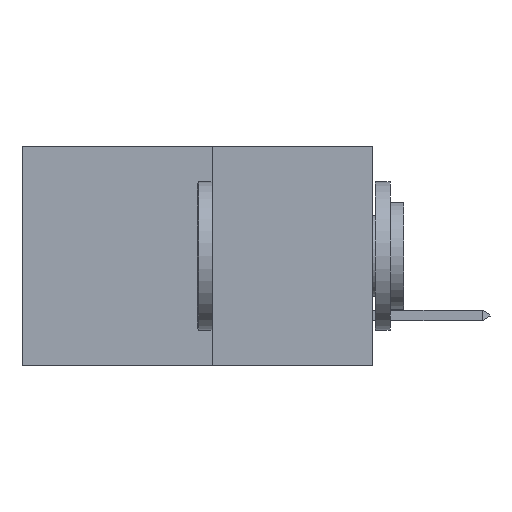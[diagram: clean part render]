
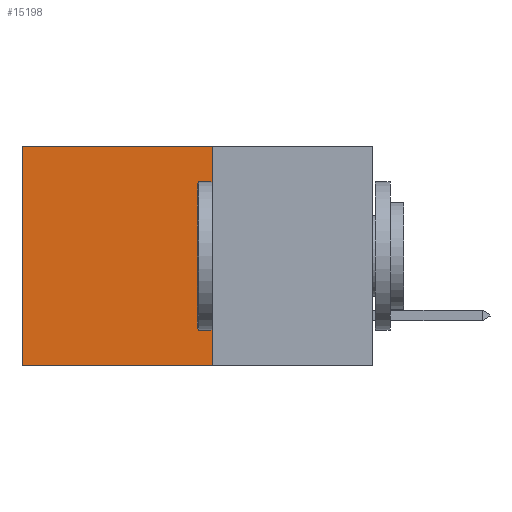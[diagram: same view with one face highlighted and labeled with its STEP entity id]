
A CAD part, left-side view. The second image highlights one B-rep face of the part: STEP entity #15198.
In plain terms, the highlighted planar face has unit normal (-1, 0, 0).
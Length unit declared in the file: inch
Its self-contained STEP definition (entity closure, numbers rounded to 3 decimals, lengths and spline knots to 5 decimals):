
#33 = LINE ( 'NONE', #5285, #3241 ) ;
#498 = ORIENTED_EDGE ( 'NONE', *, *, #5653, .F. ) ;
#578 = CARTESIAN_POINT ( 'NONE',  ( 0.277, 0.27, -0.37 ) ) ;
#868 = ORIENTED_EDGE ( 'NONE', *, *, #6116, .T. ) ;
#1072 = PLANE ( 'NONE',  #11534 ) ;
#1508 = DIRECTION ( 'NONE',  ( 0., 0., -1. ) ) ;
#1620 = CARTESIAN_POINT ( 'NONE',  ( 0.277, 0.59, -0.37 ) ) ;
#1642 = ORIENTED_EDGE ( 'NONE', *, *, #15549, .F. ) ;
#1668 = LINE ( 'NONE', #7962, #14129 ) ;
#3241 = VECTOR ( 'NONE', #5332, 39.37008 ) ;
#3577 = CARTESIAN_POINT ( 'NONE',  ( 0.277, 0.59, 0. ) ) ;
#3874 = VECTOR ( 'NONE', #11499, 39.37008 ) ;
#3959 = VERTEX_POINT ( 'NONE', #8660 ) ;
#4258 = LINE ( 'NONE', #578, #3874 ) ;
#4747 = CARTESIAN_POINT ( 'NONE',  ( 0.277, 0.27, -0.37 ) ) ;
#5165 = VECTOR ( 'NONE', #1508, 39.37008 ) ;
#5285 = CARTESIAN_POINT ( 'NONE',  ( 0.277, 0.27, -0.37 ) ) ;
#5332 = DIRECTION ( 'NONE',  ( 0., 1., 0. ) ) ;
#5653 = EDGE_CURVE ( 'NONE', #14226, #7615, #33, .T. ) ;
#5935 = FACE_OUTER_BOUND ( 'NONE', #11960, .T. ) ;
#5946 = DIRECTION ( 'NONE',  ( 0., 0., -1. ) ) ;
#6116 = EDGE_CURVE ( 'NONE', #11412, #7615, #8433, .T. ) ;
#7615 = VERTEX_POINT ( 'NONE', #8555 ) ;
#7962 = CARTESIAN_POINT ( 'NONE',  ( 0.277, 0.27, 0. ) ) ;
#8433 = LINE ( 'NONE', #1620, #5165 ) ;
#8555 = CARTESIAN_POINT ( 'NONE',  ( 0.277, 0.59, -0.37 ) ) ;
#8659 = CARTESIAN_POINT ( 'NONE',  ( 0.277, 0.27, -0.37 ) ) ;
#8660 = CARTESIAN_POINT ( 'NONE',  ( 0.277, 0.27, 0. ) ) ;
#9209 = DIRECTION ( 'NONE',  ( 0., 1., 0. ) ) ;
#10470 = EDGE_CURVE ( 'NONE', #3959, #11412, #1668, .T. ) ;
#10568 = ORIENTED_EDGE ( 'NONE', *, *, #10470, .T. ) ;
#11412 = VERTEX_POINT ( 'NONE', #3577 ) ;
#11499 = DIRECTION ( 'NONE',  ( 0., 0., -1. ) ) ;
#11534 = AXIS2_PLACEMENT_3D ( 'NONE', #4747, #13252, #5946 ) ;
#11960 = EDGE_LOOP ( 'NONE', ( #868, #498, #1642, #10568 ) ) ;
#13252 = DIRECTION ( 'NONE',  ( 1., 0., 0. ) ) ;
#14129 = VECTOR ( 'NONE', #9209, 39.37008 ) ;
#14226 = VERTEX_POINT ( 'NONE', #8659 ) ;
#15198 = ADVANCED_FACE ( 'NONE', ( #5935 ), #1072, .F. ) ;
#15549 = EDGE_CURVE ( 'NONE', #3959, #14226, #4258, .T. ) ;
